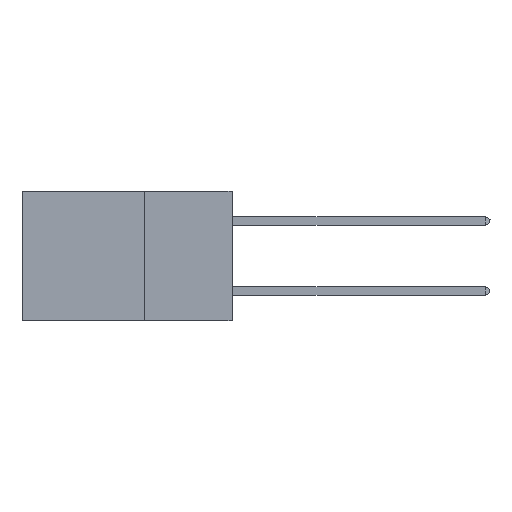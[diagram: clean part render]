
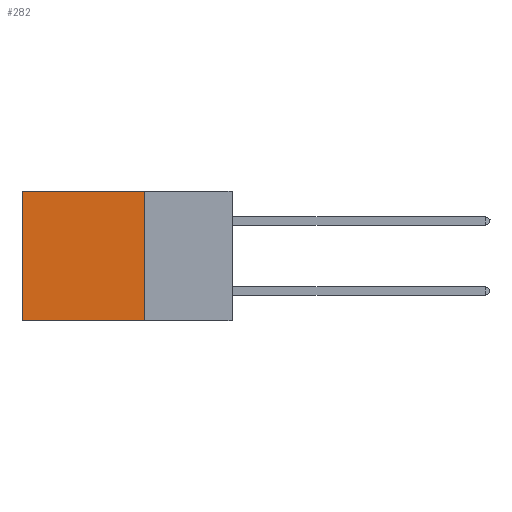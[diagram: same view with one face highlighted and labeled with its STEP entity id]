
A CAD part, left-side view. The second image highlights one B-rep face of the part: STEP entity #282.
In plain terms, the highlighted planar face has unit normal (-1, 0, 0).
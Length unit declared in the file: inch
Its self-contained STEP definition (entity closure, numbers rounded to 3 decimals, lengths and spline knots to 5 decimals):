
#282 = ADVANCED_FACE ( 'NONE', ( #34564 ), #10232, .F. ) ;
#898 = DIRECTION ( 'NONE',  ( 0., 1., 0. ) ) ;
#2447 = VECTOR ( 'NONE', #32709, 39.37008 ) ;
#2744 = CARTESIAN_POINT ( 'NONE',  ( 0.2875, 0.25, -0.37 ) ) ;
#4677 = ORIENTED_EDGE ( 'NONE', *, *, #31420, .T. ) ;
#5501 = VECTOR ( 'NONE', #25556, 39.37008 ) ;
#7627 = EDGE_CURVE ( 'NONE', #27103, #10152, #19744, .T. ) ;
#8780 = VECTOR ( 'NONE', #22582, 39.37008 ) ;
#9501 = CARTESIAN_POINT ( 'NONE',  ( 0.2875, 0.25, 0. ) ) ;
#10152 = VERTEX_POINT ( 'NONE', #27972 ) ;
#10232 = PLANE ( 'NONE',  #17898 ) ;
#11986 = LINE ( 'NONE', #28277, #8780 ) ;
#12247 = VECTOR ( 'NONE', #898, 39.37008 ) ;
#12990 = ORIENTED_EDGE ( 'NONE', *, *, #7627, .T. ) ;
#13946 = CARTESIAN_POINT ( 'NONE',  ( 0.2875, 0.25, 0. ) ) ;
#15191 = CARTESIAN_POINT ( 'NONE',  ( 0.2875, 0.6, 0. ) ) ;
#15502 = VERTEX_POINT ( 'NONE', #25650 ) ;
#16583 = ORIENTED_EDGE ( 'NONE', *, *, #21973, .F. ) ;
#17898 = AXIS2_PLACEMENT_3D ( 'NONE', #32215, #29192, #35280 ) ;
#19360 = LINE ( 'NONE', #13946, #2447 ) ;
#19744 = LINE ( 'NONE', #9501, #12247 ) ;
#20990 = CARTESIAN_POINT ( 'NONE',  ( 0.2875, 0.25, 0. ) ) ;
#21973 = EDGE_CURVE ( 'NONE', #32134, #15502, #11986, .T. ) ;
#22281 = EDGE_CURVE ( 'NONE', #27103, #32134, #19360, .T. ) ;
#22582 = DIRECTION ( 'NONE',  ( 0., 1., 0. ) ) ;
#22886 = LINE ( 'NONE', #15191, #5501 ) ;
#25556 = DIRECTION ( 'NONE',  ( 0., 0., -1. ) ) ;
#25650 = CARTESIAN_POINT ( 'NONE',  ( 0.2875, 0.6, -0.37 ) ) ;
#27103 = VERTEX_POINT ( 'NONE', #20990 ) ;
#27972 = CARTESIAN_POINT ( 'NONE',  ( 0.2875, 0.6, 0. ) ) ;
#28277 = CARTESIAN_POINT ( 'NONE',  ( 0.2875, 0.25, -0.37 ) ) ;
#29192 = DIRECTION ( 'NONE',  ( 1., 0., 0. ) ) ;
#30727 = EDGE_LOOP ( 'NONE', ( #4677, #16583, #31630, #12990 ) ) ;
#31420 = EDGE_CURVE ( 'NONE', #10152, #15502, #22886, .T. ) ;
#31630 = ORIENTED_EDGE ( 'NONE', *, *, #22281, .F. ) ;
#32134 = VERTEX_POINT ( 'NONE', #2744 ) ;
#32215 = CARTESIAN_POINT ( 'NONE',  ( 0.2875, 0.25, 0. ) ) ;
#32709 = DIRECTION ( 'NONE',  ( 0., 0., -1. ) ) ;
#34564 = FACE_OUTER_BOUND ( 'NONE', #30727, .T. ) ;
#35280 = DIRECTION ( 'NONE',  ( 0., 0., -1. ) ) ;
